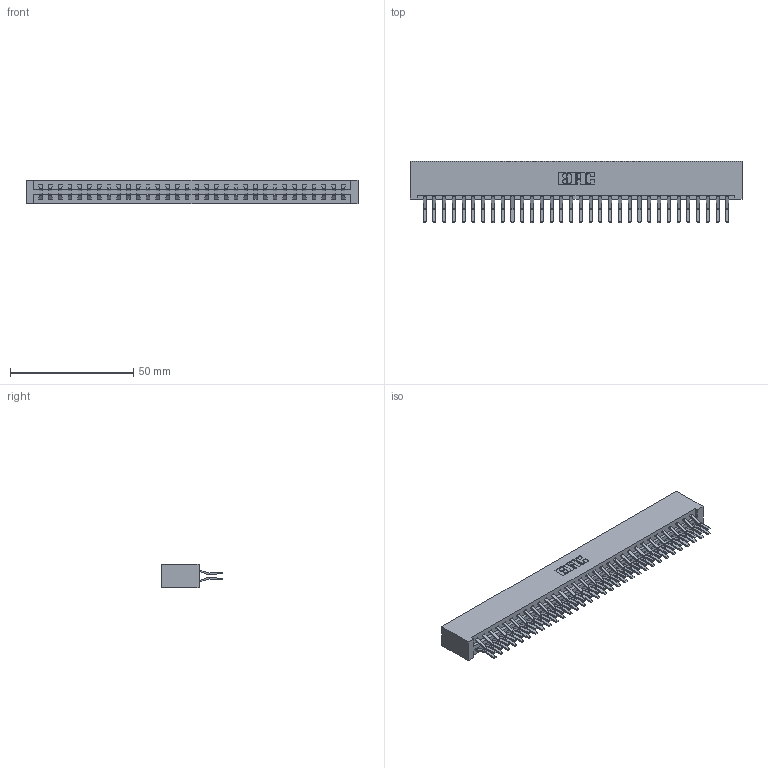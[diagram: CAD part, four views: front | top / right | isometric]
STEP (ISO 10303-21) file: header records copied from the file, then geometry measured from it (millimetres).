
FILE_DESCRIPTION (( 'STEP AP203' ), '1' );
FILE_NAME ('337-064-560-201.STEP', '2018-08-11T06:55:06', ( '' ), ( '' ), 'SwSTEP 2.0', 'SolidWorks 2016', '' );
FILE_SCHEMA (( 'CONFIG_CONTROL_DESIGN' ));
Length unit declared in the file: inch
Products named in the file (3): 337 Part_No Mounting Lugs; 345-292-001_560 Tail; 337-064-560-201
Assembly tree (65 placements, depth 2):
  337-064-560-201
    337 Part_No Mounting Lugs
    345-292-001_560 Tail  x64
Bounding box: 134.67 x 24.78 x 9.4 mm (x, y, z)
Volume: 15239.8 mm3; surface area: 18401.7 mm2
Topology: 65 solids, 65 shells, 3690 faces, 10975 edges, 7230 vertices
Faces by surface type: plane 2498, cylinder 1192
Entity records: 25915 total; most frequent: CARTESIAN_POINT 4374, ORIENTED_EDGE 4310, DIRECTION 3735, EDGE_CURVE 2155, VECTOR 2031, LINE 2031, VERTEX_POINT 1434, AXIS2_PLACEMENT_3D 852
